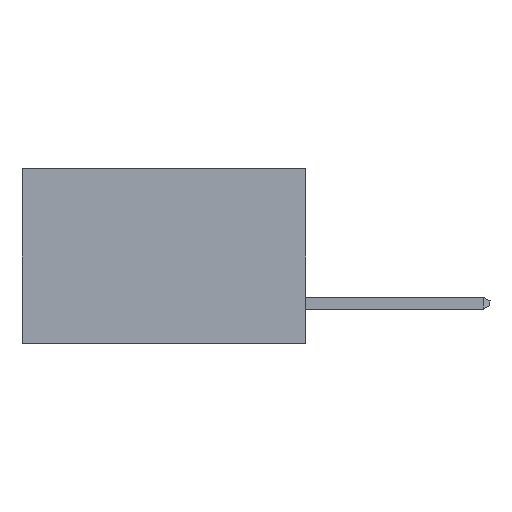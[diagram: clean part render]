
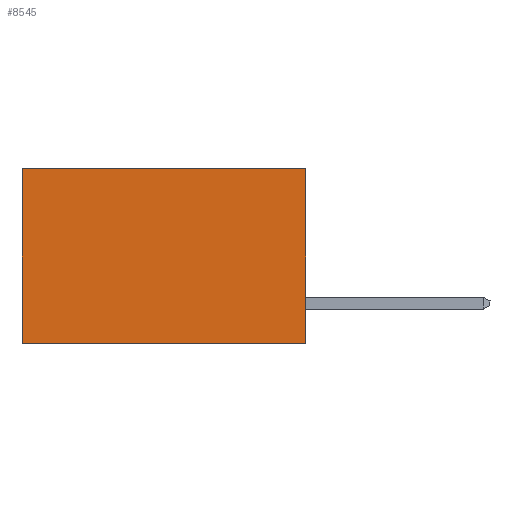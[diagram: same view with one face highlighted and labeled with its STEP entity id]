
A CAD part, left-side view. The second image highlights one B-rep face of the part: STEP entity #8545.
In plain terms, the highlighted planar face has unit normal (-1, 0, 0).
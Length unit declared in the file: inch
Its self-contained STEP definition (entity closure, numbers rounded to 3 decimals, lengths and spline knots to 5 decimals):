
#556 = VERTEX_POINT ( 'NONE', #6245 ) ;
#1075 = PLANE ( 'NONE',  #5051 ) ;
#1420 = EDGE_LOOP ( 'NONE', ( #5316, #12255, #11170, #7883 ) ) ;
#2053 = CARTESIAN_POINT ( 'NONE',  ( 0.2615, 0., 0. ) ) ;
#2146 = LINE ( 'NONE', #3431, #11435 ) ;
#2562 = CARTESIAN_POINT ( 'NONE',  ( 0.2615, 0., -0.37 ) ) ;
#2982 = VECTOR ( 'NONE', #7673, 39.37008 ) ;
#3406 = FACE_OUTER_BOUND ( 'NONE', #1420, .T. ) ;
#3431 = CARTESIAN_POINT ( 'NONE',  ( 0.2615, 0., 0. ) ) ;
#3486 = CARTESIAN_POINT ( 'NONE',  ( 0.2615, 0., -0.37 ) ) ;
#3876 = VERTEX_POINT ( 'NONE', #2053 ) ;
#3931 = DIRECTION ( 'NONE',  ( 0., 1., 0. ) ) ;
#4192 = CARTESIAN_POINT ( 'NONE',  ( 0.2615, 0., -0.37 ) ) ;
#4502 = EDGE_CURVE ( 'NONE', #9326, #556, #13814, .T. ) ;
#5051 = AXIS2_PLACEMENT_3D ( 'NONE', #3486, #8276, #13135 ) ;
#5316 = ORIENTED_EDGE ( 'NONE', *, *, #4502, .T. ) ;
#6120 = EDGE_CURVE ( 'NONE', #10430, #556, #15009, .T. ) ;
#6245 = CARTESIAN_POINT ( 'NONE',  ( 0.2615, 0.6, -0.37 ) ) ;
#6711 = VECTOR ( 'NONE', #10562, 39.37008 ) ;
#7179 = CARTESIAN_POINT ( 'NONE',  ( 0.2615, 0.6, 0. ) ) ;
#7673 = DIRECTION ( 'NONE',  ( 0., 0., -1. ) ) ;
#7883 = ORIENTED_EDGE ( 'NONE', *, *, #9177, .T. ) ;
#8276 = DIRECTION ( 'NONE',  ( 1., 0., 0. ) ) ;
#8545 = ADVANCED_FACE ( 'NONE', ( #3406 ), #1075, .F. ) ;
#9177 = EDGE_CURVE ( 'NONE', #3876, #9326, #2146, .T. ) ;
#9326 = VERTEX_POINT ( 'NONE', #7179 ) ;
#10296 = CARTESIAN_POINT ( 'NONE',  ( 0.2615, 0.6, -0.37 ) ) ;
#10370 = DIRECTION ( 'NONE',  ( 0., 1., 0. ) ) ;
#10430 = VERTEX_POINT ( 'NONE', #4192 ) ;
#10562 = DIRECTION ( 'NONE',  ( 0., 0., -1. ) ) ;
#11170 = ORIENTED_EDGE ( 'NONE', *, *, #15435, .F. ) ;
#11435 = VECTOR ( 'NONE', #10370, 39.37008 ) ;
#11832 = LINE ( 'NONE', #15438, #6711 ) ;
#12255 = ORIENTED_EDGE ( 'NONE', *, *, #6120, .F. ) ;
#13135 = DIRECTION ( 'NONE',  ( 0., 0., -1. ) ) ;
#13153 = VECTOR ( 'NONE', #3931, 39.37008 ) ;
#13814 = LINE ( 'NONE', #10296, #2982 ) ;
#15009 = LINE ( 'NONE', #2562, #13153 ) ;
#15435 = EDGE_CURVE ( 'NONE', #3876, #10430, #11832, .T. ) ;
#15438 = CARTESIAN_POINT ( 'NONE',  ( 0.2615, 0., -0.37 ) ) ;
